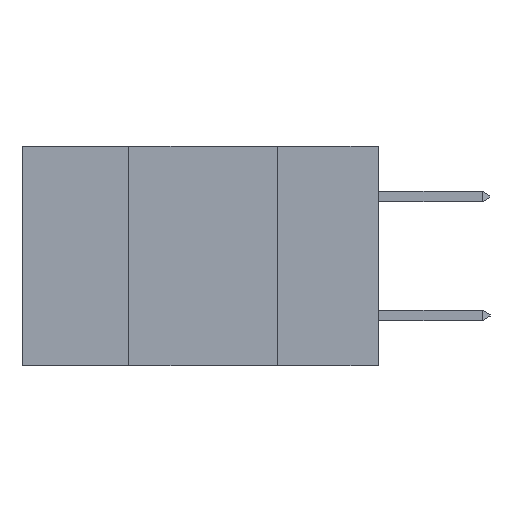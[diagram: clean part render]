
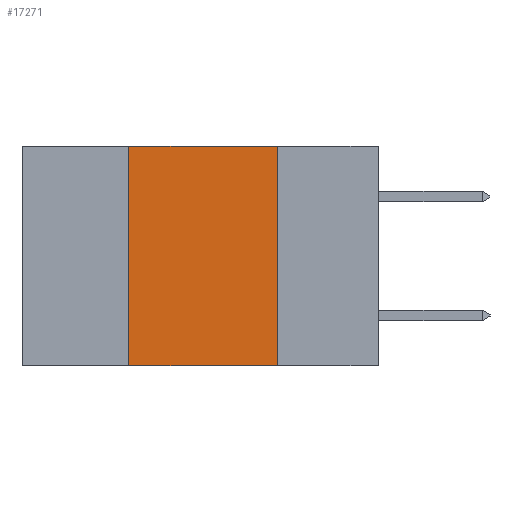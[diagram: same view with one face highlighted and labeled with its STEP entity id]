
A CAD part, left-side view. The second image highlights one B-rep face of the part: STEP entity #17271.
In plain terms, the highlighted planar face has unit normal (-1, 0, 0).
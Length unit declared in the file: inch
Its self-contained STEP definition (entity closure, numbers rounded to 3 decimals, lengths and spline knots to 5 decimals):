
#1055 = CARTESIAN_POINT ( 'NONE',  ( 0., 0.42, -0.37 ) ) ;
#1116 = ORIENTED_EDGE ( 'NONE', *, *, #1383, .T. ) ;
#1326 = AXIS2_PLACEMENT_3D ( 'NONE', #1658, #15358, #6365 ) ;
#1383 = EDGE_CURVE ( 'NONE', #11837, #8255, #11498, .T. ) ;
#1647 = CARTESIAN_POINT ( 'NONE',  ( 0., 0.42, -0.37 ) ) ;
#1658 = CARTESIAN_POINT ( 'NONE',  ( 0., 0.6, 0. ) ) ;
#1700 = VERTEX_POINT ( 'NONE', #5691 ) ;
#2888 = VECTOR ( 'NONE', #7396, 39.37008 ) ;
#2906 = VECTOR ( 'NONE', #18862, 39.37008 ) ;
#3220 = CARTESIAN_POINT ( 'NONE',  ( 0., 0.17, -0.37 ) ) ;
#5691 = CARTESIAN_POINT ( 'NONE',  ( 0., 0.17, 0. ) ) ;
#5985 = EDGE_LOOP ( 'NONE', ( #18425, #8600, #18875, #1116 ) ) ;
#6365 = DIRECTION ( 'NONE',  ( 0., 0., -1. ) ) ;
#7367 = EDGE_CURVE ( 'NONE', #11837, #16817, #13436, .T. ) ;
#7396 = DIRECTION ( 'NONE',  ( 0., -1., 0. ) ) ;
#8255 = VERTEX_POINT ( 'NONE', #3220 ) ;
#8600 = ORIENTED_EDGE ( 'NONE', *, *, #18420, .F. ) ;
#8623 = CARTESIAN_POINT ( 'NONE',  ( 0., 0.6, -0.37 ) ) ;
#9308 = VECTOR ( 'NONE', #17693, 39.37008 ) ;
#9423 = VECTOR ( 'NONE', #11863, 39.37008 ) ;
#11498 = LINE ( 'NONE', #8623, #2906 ) ;
#11837 = VERTEX_POINT ( 'NONE', #1647 ) ;
#11863 = DIRECTION ( 'NONE',  ( 0., 0., 1. ) ) ;
#12354 = PLANE ( 'NONE',  #1326 ) ;
#12904 = CARTESIAN_POINT ( 'NONE',  ( 0., 0.42, 0. ) ) ;
#13313 = LINE ( 'NONE', #14710, #9308 ) ;
#13436 = LINE ( 'NONE', #1055, #9423 ) ;
#14710 = CARTESIAN_POINT ( 'NONE',  ( 0., 0.17, -0.37 ) ) ;
#14973 = LINE ( 'NONE', #17832, #2888 ) ;
#15358 = DIRECTION ( 'NONE',  ( 1., 0., 0. ) ) ;
#16817 = VERTEX_POINT ( 'NONE', #12904 ) ;
#17271 = ADVANCED_FACE ( 'NONE', ( #18395 ), #12354, .F. ) ;
#17693 = DIRECTION ( 'NONE',  ( 0., 0., -1. ) ) ;
#17832 = CARTESIAN_POINT ( 'NONE',  ( 0., 0.6, 0. ) ) ;
#18395 = FACE_OUTER_BOUND ( 'NONE', #5985, .T. ) ;
#18420 = EDGE_CURVE ( 'NONE', #16817, #1700, #14973, .T. ) ;
#18425 = ORIENTED_EDGE ( 'NONE', *, *, #19163, .F. ) ;
#18862 = DIRECTION ( 'NONE',  ( 0., -1., 0. ) ) ;
#18875 = ORIENTED_EDGE ( 'NONE', *, *, #7367, .F. ) ;
#19163 = EDGE_CURVE ( 'NONE', #1700, #8255, #13313, .T. ) ;
